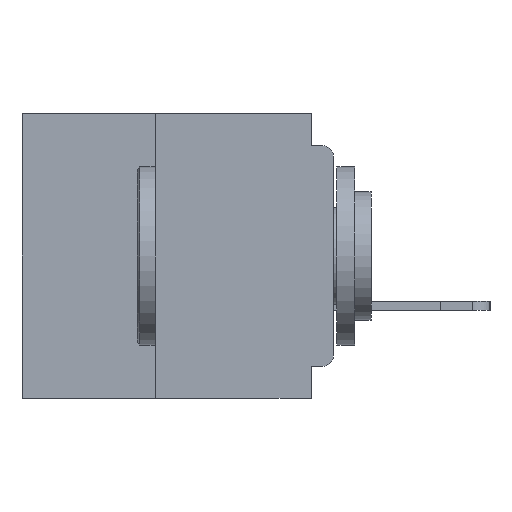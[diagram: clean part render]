
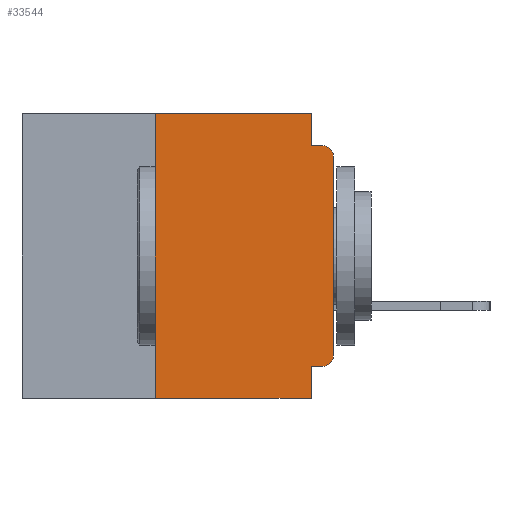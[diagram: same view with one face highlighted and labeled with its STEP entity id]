
A CAD part, left-side view. The second image highlights one B-rep face of the part: STEP entity #33544.
In plain terms, the highlighted planar face has unit normal (-1, 0, 0).
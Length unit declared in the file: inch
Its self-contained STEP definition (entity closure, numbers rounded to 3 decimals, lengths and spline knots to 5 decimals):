
#97 = VECTOR ( 'NONE', #33013, 39.37008 ) ;
#429 = DIRECTION ( 'NONE',  ( -1., 0., 0. ) ) ;
#619 = VECTOR ( 'NONE', #8913, 39.37008 ) ;
#1270 = ORIENTED_EDGE ( 'NONE', *, *, #3644, .T. ) ;
#1296 = LINE ( 'NONE', #45737, #29821 ) ;
#1604 = DIRECTION ( 'NONE',  ( 0., -1., 0. ) ) ;
#2559 = CIRCLE ( 'NONE', #44012, 0.015 ) ;
#3644 = EDGE_CURVE ( 'NONE', #43281, #20343, #7173, .T. ) ;
#4317 = LINE ( 'NONE', #34592, #13844 ) ;
#5344 = CARTESIAN_POINT ( 'NONE',  ( 0., 0., 0. ) ) ;
#5683 = CARTESIAN_POINT ( 'NONE',  ( 0., 0.015, -0.355 ) ) ;
#6605 = CARTESIAN_POINT ( 'NONE',  ( 0., 0., -0.045 ) ) ;
#7088 = CARTESIAN_POINT ( 'NONE',  ( 0., 0.015, -0.06 ) ) ;
#7173 = LINE ( 'NONE', #23003, #34573 ) ;
#8005 = CARTESIAN_POINT ( 'NONE',  ( 0., 0.031, -0.4 ) ) ;
#8473 = LINE ( 'NONE', #8005, #97 ) ;
#8913 = DIRECTION ( 'NONE',  ( 0., 0., 1. ) ) ;
#10488 = CARTESIAN_POINT ( 'NONE',  ( 0., 0.031, -0.355 ) ) ;
#10679 = DIRECTION ( 'NONE',  ( 0., 0., -1. ) ) ;
#10869 = CARTESIAN_POINT ( 'NONE',  ( 0., 0.437, 0. ) ) ;
#11506 = ORIENTED_EDGE ( 'NONE', *, *, #23664, .F. ) ;
#13479 = EDGE_CURVE ( 'NONE', #26587, #26498, #21433, .T. ) ;
#13630 = ORIENTED_EDGE ( 'NONE', *, *, #21567, .F. ) ;
#13844 = VECTOR ( 'NONE', #27242, 39.37008 ) ;
#14459 = DIRECTION ( 'NONE',  ( 0., 0., -1. ) ) ;
#16498 = CARTESIAN_POINT ( 'NONE',  ( 0., 0.015, -0.045 ) ) ;
#16919 = DIRECTION ( 'NONE',  ( 0., -1., 0. ) ) ;
#17385 = DIRECTION ( 'NONE',  ( 0., -1., 0. ) ) ;
#17521 = EDGE_CURVE ( 'NONE', #26545, #20907, #2559, .T. ) ;
#18119 = CARTESIAN_POINT ( 'NONE',  ( 0., 0.031, 0. ) ) ;
#18911 = LINE ( 'NONE', #6605, #36829 ) ;
#19400 = CARTESIAN_POINT ( 'NONE',  ( 0., 0.25, -0.4 ) ) ;
#19831 = CARTESIAN_POINT ( 'NONE',  ( 0., 0.031, -0.4 ) ) ;
#20343 = VERTEX_POINT ( 'NONE', #19831 ) ;
#20907 = VERTEX_POINT ( 'NONE', #16498 ) ;
#21433 = CIRCLE ( 'NONE', #32525, 0.015 ) ;
#21534 = VERTEX_POINT ( 'NONE', #34280 ) ;
#21567 = EDGE_CURVE ( 'NONE', #26587, #38311, #4317, .T. ) ;
#21838 = CARTESIAN_POINT ( 'NONE',  ( 0., 0.015, -0.34 ) ) ;
#22945 = CARTESIAN_POINT ( 'NONE',  ( 0., 0.25, -0.4 ) ) ;
#23003 = CARTESIAN_POINT ( 'NONE',  ( 0., 0.437, -0.4 ) ) ;
#23664 = EDGE_CURVE ( 'NONE', #43281, #41954, #32173, .T. ) ;
#25052 = PLANE ( 'NONE',  #42175 ) ;
#25387 = DIRECTION ( 'NONE',  ( 0., 0., -1. ) ) ;
#25958 = FACE_OUTER_BOUND ( 'NONE', #43623, .T. ) ;
#26498 = VERTEX_POINT ( 'NONE', #30223 ) ;
#26545 = VERTEX_POINT ( 'NONE', #41171 ) ;
#26587 = VERTEX_POINT ( 'NONE', #5683 ) ;
#26651 = EDGE_CURVE ( 'NONE', #41954, #36666, #41296, .T. ) ;
#26735 = EDGE_CURVE ( 'NONE', #21534, #20907, #18911, .T. ) ;
#27242 = DIRECTION ( 'NONE',  ( 0., 1., 0. ) ) ;
#28711 = ORIENTED_EDGE ( 'NONE', *, *, #13479, .T. ) ;
#29135 = LINE ( 'NONE', #5344, #619 ) ;
#29401 = ORIENTED_EDGE ( 'NONE', *, *, #30180, .F. ) ;
#29821 = VECTOR ( 'NONE', #31336, 39.37008 ) ;
#30180 = EDGE_CURVE ( 'NONE', #36666, #21534, #1296, .T. ) ;
#30223 = CARTESIAN_POINT ( 'NONE',  ( 0., 0., -0.34 ) ) ;
#30669 = VECTOR ( 'NONE', #16919, 39.37008 ) ;
#30698 = ORIENTED_EDGE ( 'NONE', *, *, #26735, .F. ) ;
#31336 = DIRECTION ( 'NONE',  ( 0., 0., -1. ) ) ;
#32105 = DIRECTION ( 'NONE',  ( -1., 0., 0. ) ) ;
#32173 = LINE ( 'NONE', #19400, #40529 ) ;
#32525 = AXIS2_PLACEMENT_3D ( 'NONE', #21838, #429, #25387 ) ;
#33013 = DIRECTION ( 'NONE',  ( 0., 0., -1. ) ) ;
#33159 = ORIENTED_EDGE ( 'NONE', *, *, #17521, .T. ) ;
#33544 = ADVANCED_FACE ( 'NONE', ( #25958 ), #25052, .F. ) ;
#34280 = CARTESIAN_POINT ( 'NONE',  ( 0., 0.031, -0.045 ) ) ;
#34573 = VECTOR ( 'NONE', #1604, 39.37008 ) ;
#34592 = CARTESIAN_POINT ( 'NONE',  ( 0., 0., -0.355 ) ) ;
#35876 = DIRECTION ( 'NONE',  ( 1., 0., 0. ) ) ;
#36091 = EDGE_CURVE ( 'NONE', #38311, #20343, #8473, .T. ) ;
#36258 = EDGE_CURVE ( 'NONE', #26498, #26545, #29135, .T. ) ;
#36666 = VERTEX_POINT ( 'NONE', #18119 ) ;
#36829 = VECTOR ( 'NONE', #17385, 39.37008 ) ;
#36985 = ORIENTED_EDGE ( 'NONE', *, *, #36091, .F. ) ;
#37972 = ORIENTED_EDGE ( 'NONE', *, *, #36258, .T. ) ;
#38311 = VERTEX_POINT ( 'NONE', #10488 ) ;
#38350 = CARTESIAN_POINT ( 'NONE',  ( 0., 0.437, 0. ) ) ;
#40529 = VECTOR ( 'NONE', #40819, 39.37008 ) ;
#40819 = DIRECTION ( 'NONE',  ( 0., 0., 1. ) ) ;
#41171 = CARTESIAN_POINT ( 'NONE',  ( 0., 0., -0.06 ) ) ;
#41296 = LINE ( 'NONE', #38350, #30669 ) ;
#41954 = VERTEX_POINT ( 'NONE', #43539 ) ;
#42175 = AXIS2_PLACEMENT_3D ( 'NONE', #10869, #35876, #14459 ) ;
#43281 = VERTEX_POINT ( 'NONE', #22945 ) ;
#43539 = CARTESIAN_POINT ( 'NONE',  ( 0., 0.25, 0. ) ) ;
#43623 = EDGE_LOOP ( 'NONE', ( #37972, #33159, #30698, #29401, #46200, #11506, #1270, #36985, #13630, #28711 ) ) ;
#44012 = AXIS2_PLACEMENT_3D ( 'NONE', #7088, #32105, #10679 ) ;
#45737 = CARTESIAN_POINT ( 'NONE',  ( 0., 0.031, 0. ) ) ;
#46200 = ORIENTED_EDGE ( 'NONE', *, *, #26651, .F. ) ;
